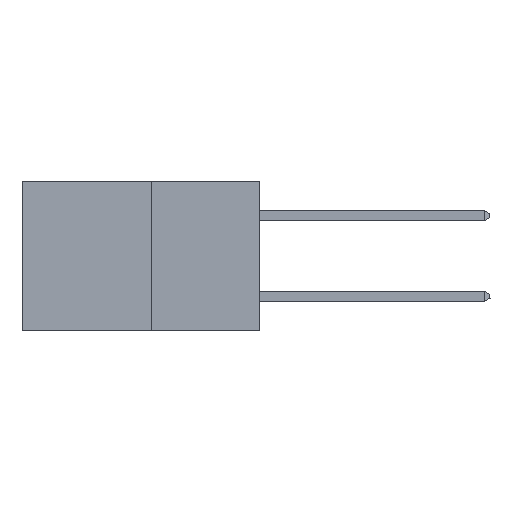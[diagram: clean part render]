
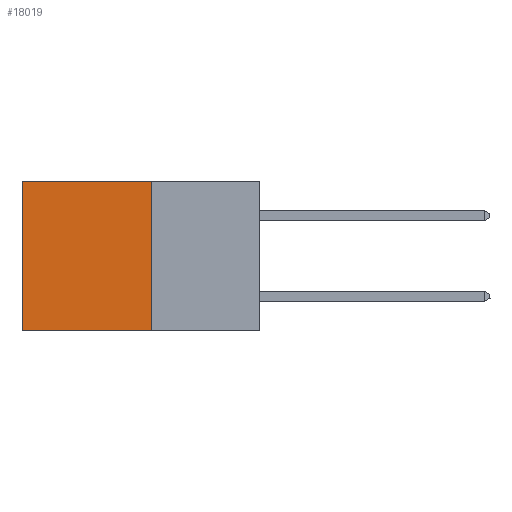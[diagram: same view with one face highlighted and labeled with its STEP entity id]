
A CAD part, left-side view. The second image highlights one B-rep face of the part: STEP entity #18019.
In plain terms, the highlighted planar face has unit normal (-1, 0, 0).
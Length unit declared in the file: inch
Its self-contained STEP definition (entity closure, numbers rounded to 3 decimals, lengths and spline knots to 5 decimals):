
#411 = DIRECTION ( 'NONE',  ( 0., 1., 0. ) ) ;
#1604 = EDGE_CURVE ( 'NONE', #25536, #13910, #1978, .T. ) ;
#1978 = LINE ( 'NONE', #11947, #3282 ) ;
#2030 = VECTOR ( 'NONE', #411, 39.37008 ) ;
#2437 = EDGE_CURVE ( 'NONE', #12296, #11517, #8827, .T. ) ;
#2731 = EDGE_CURVE ( 'NONE', #12296, #25536, #7823, .T. ) ;
#3282 = VECTOR ( 'NONE', #4635, 39.37008 ) ;
#4635 = DIRECTION ( 'NONE',  ( 0., 0., -1. ) ) ;
#5238 = DIRECTION ( 'NONE',  ( 1., 0., 0. ) ) ;
#7606 = LINE ( 'NONE', #19193, #2030 ) ;
#7823 = LINE ( 'NONE', #21605, #18232 ) ;
#8827 = LINE ( 'NONE', #12812, #13708 ) ;
#10364 = CARTESIAN_POINT ( 'NONE',  ( 0.277, 0.59, 0. ) ) ;
#10495 = ORIENTED_EDGE ( 'NONE', *, *, #24335, .F. ) ;
#10933 = DIRECTION ( 'NONE',  ( 0., 1., 0. ) ) ;
#11517 = VERTEX_POINT ( 'NONE', #22197 ) ;
#11947 = CARTESIAN_POINT ( 'NONE',  ( 0.277, 0.59, -0.37 ) ) ;
#12296 = VERTEX_POINT ( 'NONE', #24676 ) ;
#12812 = CARTESIAN_POINT ( 'NONE',  ( 0.277, 0.27, -0.37 ) ) ;
#13050 = CARTESIAN_POINT ( 'NONE',  ( 0.277, 0.59, -0.37 ) ) ;
#13474 = CARTESIAN_POINT ( 'NONE',  ( 0.277, 0.27, -0.37 ) ) ;
#13708 = VECTOR ( 'NONE', #17442, 39.37008 ) ;
#13910 = VERTEX_POINT ( 'NONE', #13050 ) ;
#14778 = EDGE_LOOP ( 'NONE', ( #16388, #10495, #26743, #17642 ) ) ;
#16388 = ORIENTED_EDGE ( 'NONE', *, *, #1604, .T. ) ;
#17442 = DIRECTION ( 'NONE',  ( 0., 0., -1. ) ) ;
#17642 = ORIENTED_EDGE ( 'NONE', *, *, #2731, .T. ) ;
#18019 = ADVANCED_FACE ( 'NONE', ( #20668 ), #25903, .F. ) ;
#18232 = VECTOR ( 'NONE', #10933, 39.37008 ) ;
#19193 = CARTESIAN_POINT ( 'NONE',  ( 0.277, 0.27, -0.37 ) ) ;
#19754 = DIRECTION ( 'NONE',  ( 0., 0., -1. ) ) ;
#20668 = FACE_OUTER_BOUND ( 'NONE', #14778, .T. ) ;
#21432 = AXIS2_PLACEMENT_3D ( 'NONE', #13474, #5238, #19754 ) ;
#21605 = CARTESIAN_POINT ( 'NONE',  ( 0.277, 0.27, 0. ) ) ;
#22197 = CARTESIAN_POINT ( 'NONE',  ( 0.277, 0.27, -0.37 ) ) ;
#24335 = EDGE_CURVE ( 'NONE', #11517, #13910, #7606, .T. ) ;
#24676 = CARTESIAN_POINT ( 'NONE',  ( 0.277, 0.27, 0. ) ) ;
#25536 = VERTEX_POINT ( 'NONE', #10364 ) ;
#25903 = PLANE ( 'NONE',  #21432 ) ;
#26743 = ORIENTED_EDGE ( 'NONE', *, *, #2437, .F. ) ;
